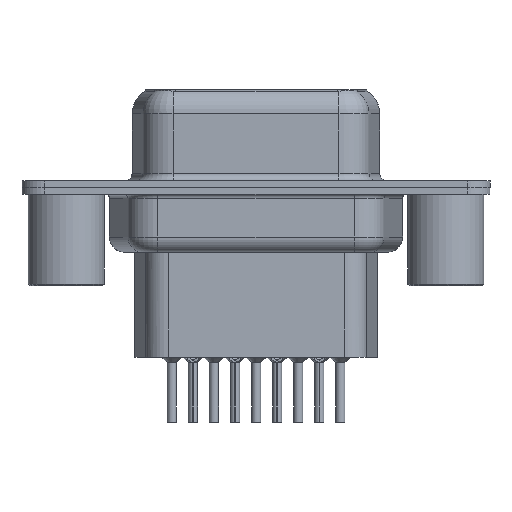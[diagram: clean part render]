
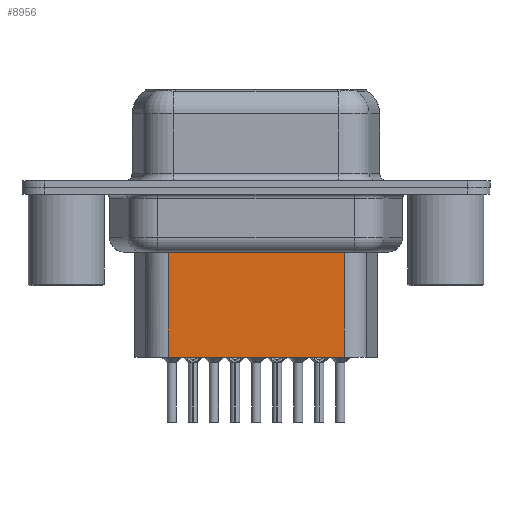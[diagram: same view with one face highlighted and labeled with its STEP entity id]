
A CAD part, front view. The second image highlights one B-rep face of the part: STEP entity #8956.
In plain terms, the highlighted planar face has unit normal (0, -1, 0).
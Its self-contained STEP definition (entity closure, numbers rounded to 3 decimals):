
#12 = DIRECTION ( 'NONE',  ( 0., 0., -1. ) ) ;
#312 = DIRECTION ( 'NONE',  ( -1., 0., 0. ) ) ;
#1653 = EDGE_CURVE ( 'NONE', #20712, #3139, #10577, .T. ) ;
#2043 = EDGE_CURVE ( 'NONE', #10603, #20712, #2257, .T. ) ;
#2194 = AXIS2_PLACEMENT_3D ( 'NONE', #9376, #17529, #16200 ) ;
#2207 = EDGE_CURVE ( 'NONE', #12582, #3139, #5279, .T. ) ;
#2257 = LINE ( 'NONE', #12519, #4440 ) ;
#2268 = CARTESIAN_POINT ( 'NONE',  ( 6.706, -3.5, -4.097 ) ) ;
#3139 = VERTEX_POINT ( 'NONE', #3759 ) ;
#3759 = CARTESIAN_POINT ( 'NONE',  ( 6.706, -3.5, -11.15 ) ) ;
#3923 = EDGE_CURVE ( 'NONE', #10603, #12582, #14176, .T. ) ;
#4440 = VECTOR ( 'NONE', #10849, 1000. ) ;
#5279 = LINE ( 'NONE', #22140, #5572 ) ;
#5572 = VECTOR ( 'NONE', #12, 1000. ) ;
#6315 = VECTOR ( 'NONE', #17510, 1000. ) ;
#8245 = EDGE_LOOP ( 'NONE', ( #17678, #10811, #10433, #12491 ) ) ;
#8956 = ADVANCED_FACE ( 'NONE', ( #14200 ), #9043, .T. ) ;
#9043 = PLANE ( 'NONE',  #2194 ) ;
#9376 = CARTESIAN_POINT ( 'NONE',  ( 6.706, -3.5, -3.1 ) ) ;
#10433 = ORIENTED_EDGE ( 'NONE', *, *, #2207, .T. ) ;
#10577 = LINE ( 'NONE', #18938, #15954 ) ;
#10603 = VERTEX_POINT ( 'NONE', #13912 ) ;
#10811 = ORIENTED_EDGE ( 'NONE', *, *, #3923, .T. ) ;
#10849 = DIRECTION ( 'NONE',  ( 0., 0., -1. ) ) ;
#12491 = ORIENTED_EDGE ( 'NONE', *, *, #1653, .F. ) ;
#12519 = CARTESIAN_POINT ( 'NONE',  ( 18.294, -3.5, -3.1 ) ) ;
#12582 = VERTEX_POINT ( 'NONE', #2268 ) ;
#13912 = CARTESIAN_POINT ( 'NONE',  ( 18.294, -3.5, -4.097 ) ) ;
#14176 = LINE ( 'NONE', #15633, #6315 ) ;
#14200 = FACE_OUTER_BOUND ( 'NONE', #8245, .T. ) ;
#15633 = CARTESIAN_POINT ( 'NONE',  ( 6.459, -3.5, -4.097 ) ) ;
#15954 = VECTOR ( 'NONE', #312, 1000. ) ;
#16200 = DIRECTION ( 'NONE',  ( 1., 0., 0. ) ) ;
#16902 = CARTESIAN_POINT ( 'NONE',  ( 18.294, -3.5, -11.15 ) ) ;
#17510 = DIRECTION ( 'NONE',  ( -1., 0., 0. ) ) ;
#17529 = DIRECTION ( 'NONE',  ( 0., -1., 0. ) ) ;
#17678 = ORIENTED_EDGE ( 'NONE', *, *, #2043, .F. ) ;
#18938 = CARTESIAN_POINT ( 'NONE',  ( 6.706, -3.5, -11.15 ) ) ;
#20712 = VERTEX_POINT ( 'NONE', #16902 ) ;
#22140 = CARTESIAN_POINT ( 'NONE',  ( 6.706, -3.5, -3.1 ) ) ;
